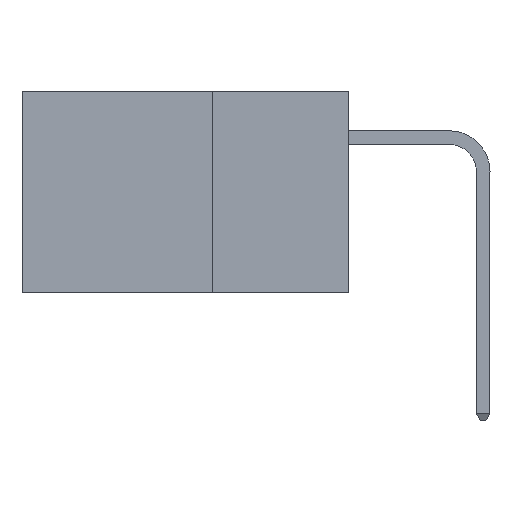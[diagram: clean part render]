
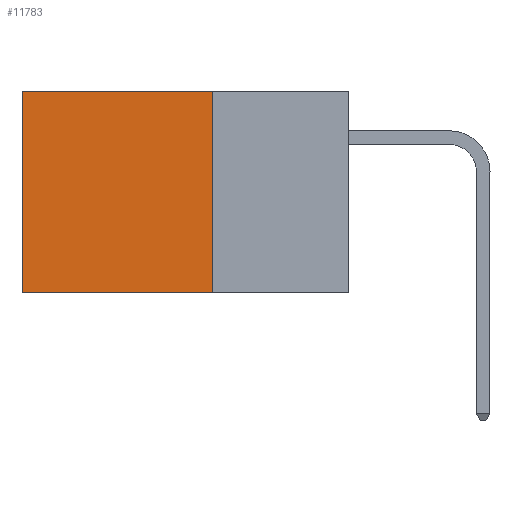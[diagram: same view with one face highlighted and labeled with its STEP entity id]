
A CAD part, left-side view. The second image highlights one B-rep face of the part: STEP entity #11783.
In plain terms, the highlighted planar face has unit normal (-1, 0, 0).
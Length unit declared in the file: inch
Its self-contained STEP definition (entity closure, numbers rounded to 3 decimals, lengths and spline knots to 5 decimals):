
#259 = ORIENTED_EDGE ( 'NONE', *, *, #10506, .F. ) ;
#581 = VECTOR ( 'NONE', #10038, 39.37008 ) ;
#1057 = CARTESIAN_POINT ( 'NONE',  ( 0.2875, 0.25, 0. ) ) ;
#1363 = CARTESIAN_POINT ( 'NONE',  ( 0.2875, 0.6, 0. ) ) ;
#1565 = VERTEX_POINT ( 'NONE', #13517 ) ;
#1777 = ORIENTED_EDGE ( 'NONE', *, *, #10859, .T. ) ;
#1835 = VECTOR ( 'NONE', #8238, 39.37008 ) ;
#1902 = CARTESIAN_POINT ( 'NONE',  ( 0.2875, 0.25, 0. ) ) ;
#2205 = DIRECTION ( 'NONE',  ( 0., 1., 0. ) ) ;
#2598 = VERTEX_POINT ( 'NONE', #1363 ) ;
#3015 = EDGE_CURVE ( 'NONE', #2598, #1565, #3992, .T. ) ;
#3101 = FACE_OUTER_BOUND ( 'NONE', #10564, .T. ) ;
#3301 = VERTEX_POINT ( 'NONE', #7080 ) ;
#3581 = CARTESIAN_POINT ( 'NONE',  ( 0.2875, 0.25, -0.37 ) ) ;
#3702 = DIRECTION ( 'NONE',  ( 0., 0., -1. ) ) ;
#3992 = LINE ( 'NONE', #6932, #1835 ) ;
#4925 = DIRECTION ( 'NONE',  ( 1., 0., 0. ) ) ;
#5708 = CARTESIAN_POINT ( 'NONE',  ( 0.2875, 0.25, 0. ) ) ;
#6932 = CARTESIAN_POINT ( 'NONE',  ( 0.2875, 0.6, 0. ) ) ;
#7080 = CARTESIAN_POINT ( 'NONE',  ( 0.2875, 0.25, -0.37 ) ) ;
#7251 = EDGE_CURVE ( 'NONE', #13164, #3301, #14502, .T. ) ;
#7996 = VECTOR ( 'NONE', #9648, 39.37008 ) ;
#8238 = DIRECTION ( 'NONE',  ( 0., 0., -1. ) ) ;
#9374 = PLANE ( 'NONE',  #14755 ) ;
#9497 = VECTOR ( 'NONE', #2205, 39.37008 ) ;
#9628 = ORIENTED_EDGE ( 'NONE', *, *, #3015, .T. ) ;
#9648 = DIRECTION ( 'NONE',  ( 0., 0., -1. ) ) ;
#10038 = DIRECTION ( 'NONE',  ( 0., 1., 0. ) ) ;
#10506 = EDGE_CURVE ( 'NONE', #3301, #1565, #12000, .T. ) ;
#10564 = EDGE_LOOP ( 'NONE', ( #9628, #259, #13150, #1777 ) ) ;
#10859 = EDGE_CURVE ( 'NONE', #13164, #2598, #15518, .T. ) ;
#11783 = ADVANCED_FACE ( 'NONE', ( #3101 ), #9374, .F. ) ;
#12000 = LINE ( 'NONE', #3581, #9497 ) ;
#13150 = ORIENTED_EDGE ( 'NONE', *, *, #7251, .F. ) ;
#13164 = VERTEX_POINT ( 'NONE', #14561 ) ;
#13517 = CARTESIAN_POINT ( 'NONE',  ( 0.2875, 0.6, -0.37 ) ) ;
#14502 = LINE ( 'NONE', #5708, #7996 ) ;
#14561 = CARTESIAN_POINT ( 'NONE',  ( 0.2875, 0.25, 0. ) ) ;
#14755 = AXIS2_PLACEMENT_3D ( 'NONE', #1902, #4925, #3702 ) ;
#15518 = LINE ( 'NONE', #1057, #581 ) ;
